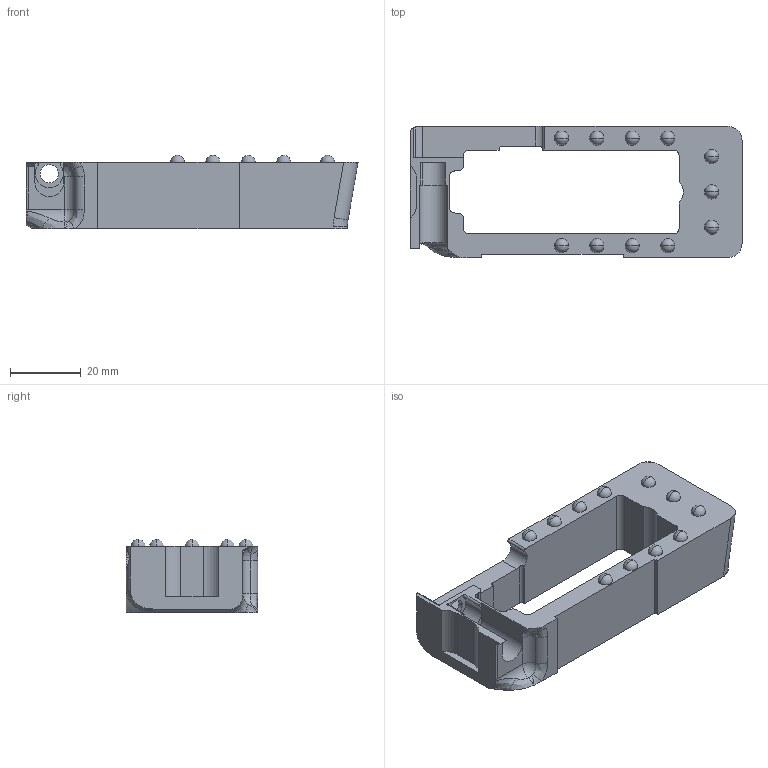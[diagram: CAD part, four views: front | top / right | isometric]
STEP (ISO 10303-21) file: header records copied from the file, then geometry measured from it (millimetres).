
FILE_DESCRIPTION (( 'STEP AP214' ), '1' );
FILE_NAME ('Magwell_2.STEP', '2015-10-23T19:41:28', ( 'WarFairy' ), ( '' ), 'SwSTEP 2.0', 'SolidWorks 2015', '' );
FILE_SCHEMA (( 'AUTOMOTIVE_DESIGN' ));
Length unit declared in the file: inch
Products named in the file (1): Magwell_2
Bounding box: 93.81 x 37.13 x 20.71 mm (x, y, z)
Volume: 30558.9 mm3; surface area: 11910.5 mm2
Topology: 1 solids, 1 shells, 123 faces, 369 edges, 236 vertices
Faces by surface type: cylinder 43, plane 34, sphere 24, bspline 15, torus 7
Entity records: 4645 total; most frequent: CARTESIAN_POINT 1573, ORIENTED_EDGE 648, DIRECTION 622, EDGE_CURVE 324, AXIS2_PLACEMENT_3D 243, VERTEX_POINT 214, EDGE_LOOP 138, LINE 136
